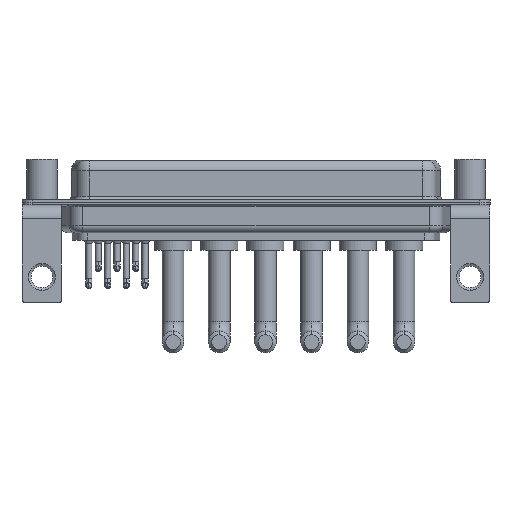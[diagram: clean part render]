
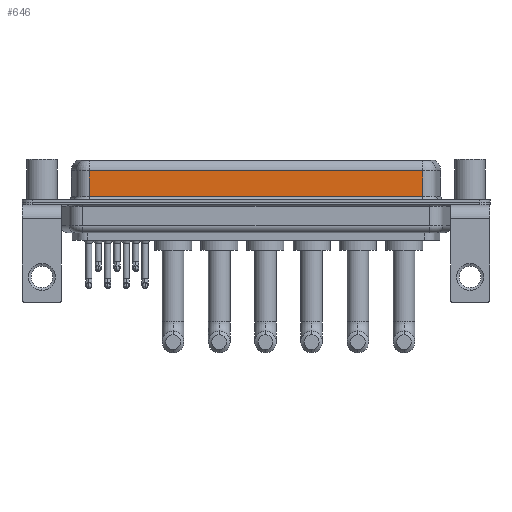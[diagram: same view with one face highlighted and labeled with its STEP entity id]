
A CAD part, front view. The second image highlights one B-rep face of the part: STEP entity #646.
In plain terms, the highlighted planar face has unit normal (0, -1, 0).
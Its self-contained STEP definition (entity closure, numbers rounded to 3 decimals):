
#151 = DIRECTION ( 'NONE',  ( 0., 0., -1. ) ) ;
#222 = ORIENTED_EDGE ( 'NONE', *, *, #18394, .F. ) ;
#646 = ADVANCED_FACE ( 'NONE', ( #17537 ), #7806, .F. ) ;
#1102 = CARTESIAN_POINT ( 'NONE',  ( 56.462, -3.95, 4.65 ) ) ;
#1345 = DIRECTION ( 'NONE',  ( 0., 0., 1. ) ) ;
#1467 = VERTEX_POINT ( 'NONE', #2726 ) ;
#2563 = LINE ( 'NONE', #1102, #8716 ) ;
#2617 = LINE ( 'NONE', #10794, #12002 ) ;
#2726 = CARTESIAN_POINT ( 'NONE',  ( 56.462, -3.95, 0.9 ) ) ;
#4333 = VERTEX_POINT ( 'NONE', #9080 ) ;
#4375 = DIRECTION ( 'NONE',  ( -1., 0., 0. ) ) ;
#6806 = VERTEX_POINT ( 'NONE', #13483 ) ;
#7806 = PLANE ( 'NONE',  #16508 ) ;
#8472 = VERTEX_POINT ( 'NONE', #9014 ) ;
#8662 = VECTOR ( 'NONE', #15447, 1000. ) ;
#8716 = VECTOR ( 'NONE', #4375, 1000. ) ;
#9014 = CARTESIAN_POINT ( 'NONE',  ( 7.038, -3.95, 4.65 ) ) ;
#9080 = CARTESIAN_POINT ( 'NONE',  ( 7.038, -3.95, 0.9 ) ) ;
#9192 = CARTESIAN_POINT ( 'NONE',  ( 56.462, -3.95, 6.4 ) ) ;
#9385 = CARTESIAN_POINT ( 'NONE',  ( 56.462, -3.95, 6.4 ) ) ;
#9586 = EDGE_CURVE ( 'NONE', #6806, #8472, #2563, .T. ) ;
#10236 = EDGE_LOOP ( 'NONE', ( #222, #14937, #13651, #19672 ) ) ;
#10794 = CARTESIAN_POINT ( 'NONE',  ( 56.462, -3.95, 0.9 ) ) ;
#11370 = CARTESIAN_POINT ( 'NONE',  ( 7.038, -3.95, 6.4 ) ) ;
#12002 = VECTOR ( 'NONE', #17254, 1000. ) ;
#13483 = CARTESIAN_POINT ( 'NONE',  ( 56.462, -3.95, 4.65 ) ) ;
#13651 = ORIENTED_EDGE ( 'NONE', *, *, #15236, .T. ) ;
#14024 = VECTOR ( 'NONE', #151, 1000. ) ;
#14063 = LINE ( 'NONE', #9192, #8662 ) ;
#14937 = ORIENTED_EDGE ( 'NONE', *, *, #9586, .T. ) ;
#15236 = EDGE_CURVE ( 'NONE', #8472, #4333, #16136, .T. ) ;
#15447 = DIRECTION ( 'NONE',  ( 0., 0., -1. ) ) ;
#15983 = EDGE_CURVE ( 'NONE', #4333, #1467, #2617, .T. ) ;
#16136 = LINE ( 'NONE', #11370, #14024 ) ;
#16508 = AXIS2_PLACEMENT_3D ( 'NONE', #9385, #20627, #1345 ) ;
#17254 = DIRECTION ( 'NONE',  ( 1., 0., 0. ) ) ;
#17537 = FACE_OUTER_BOUND ( 'NONE', #10236, .T. ) ;
#18394 = EDGE_CURVE ( 'NONE', #6806, #1467, #14063, .T. ) ;
#19672 = ORIENTED_EDGE ( 'NONE', *, *, #15983, .T. ) ;
#20627 = DIRECTION ( 'NONE',  ( 0., 1., 0. ) ) ;
